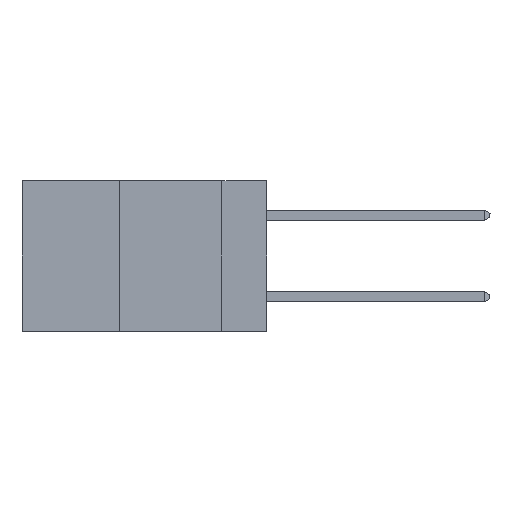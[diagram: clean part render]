
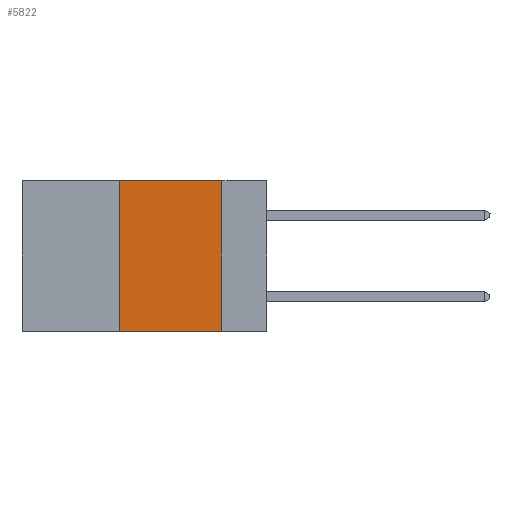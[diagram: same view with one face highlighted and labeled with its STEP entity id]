
A CAD part, left-side view. The second image highlights one B-rep face of the part: STEP entity #5822.
In plain terms, the highlighted planar face has unit normal (-1, 0, 0).
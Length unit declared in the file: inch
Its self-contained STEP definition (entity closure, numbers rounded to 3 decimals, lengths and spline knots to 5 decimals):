
#337 = DIRECTION ( 'NONE',  ( 0., -1., 0. ) ) ;
#737 = CARTESIAN_POINT ( 'NONE',  ( 0., 0.36, 0. ) ) ;
#1369 = LINE ( 'NONE', #12020, #12686 ) ;
#2554 = EDGE_CURVE ( 'NONE', #6572, #6282, #17058, .T. ) ;
#3341 = ORIENTED_EDGE ( 'NONE', *, *, #2554, .T. ) ;
#3881 = LINE ( 'NONE', #17930, #14264 ) ;
#4101 = CARTESIAN_POINT ( 'NONE',  ( 0., 0.36, 0. ) ) ;
#5822 = ADVANCED_FACE ( 'NONE', ( #9731 ), #19929, .F. ) ;
#5995 = EDGE_LOOP ( 'NONE', ( #15096, #18380, #22753, #3341 ) ) ;
#6282 = VERTEX_POINT ( 'NONE', #9473 ) ;
#6572 = VERTEX_POINT ( 'NONE', #19521 ) ;
#8205 = VECTOR ( 'NONE', #18675, 39.37008 ) ;
#8872 = EDGE_CURVE ( 'NONE', #9933, #14771, #3881, .T. ) ;
#9473 = CARTESIAN_POINT ( 'NONE',  ( 0., 0.11, -0.37 ) ) ;
#9731 = FACE_OUTER_BOUND ( 'NONE', #5995, .T. ) ;
#9933 = VERTEX_POINT ( 'NONE', #737 ) ;
#10208 = AXIS2_PLACEMENT_3D ( 'NONE', #21669, #11010, #18157 ) ;
#11010 = DIRECTION ( 'NONE',  ( 1., 0., 0. ) ) ;
#12020 = CARTESIAN_POINT ( 'NONE',  ( 0., 0.11, 0. ) ) ;
#12315 = VECTOR ( 'NONE', #20284, 39.37008 ) ;
#12686 = VECTOR ( 'NONE', #19186, 39.37008 ) ;
#13643 = CARTESIAN_POINT ( 'NONE',  ( 0., 0.6, -0.37 ) ) ;
#14264 = VECTOR ( 'NONE', #337, 39.37008 ) ;
#14379 = EDGE_CURVE ( 'NONE', #14771, #6282, #1369, .T. ) ;
#14771 = VERTEX_POINT ( 'NONE', #22022 ) ;
#15096 = ORIENTED_EDGE ( 'NONE', *, *, #14379, .F. ) ;
#17058 = LINE ( 'NONE', #13643, #8205 ) ;
#17930 = CARTESIAN_POINT ( 'NONE',  ( 0., 0.6, 0. ) ) ;
#18157 = DIRECTION ( 'NONE',  ( 0., 0., -1. ) ) ;
#18380 = ORIENTED_EDGE ( 'NONE', *, *, #8872, .F. ) ;
#18636 = LINE ( 'NONE', #4101, #12315 ) ;
#18675 = DIRECTION ( 'NONE',  ( 0., -1., 0. ) ) ;
#19186 = DIRECTION ( 'NONE',  ( 0., 0., -1. ) ) ;
#19521 = CARTESIAN_POINT ( 'NONE',  ( 0., 0.36, -0.37 ) ) ;
#19929 = PLANE ( 'NONE',  #10208 ) ;
#20284 = DIRECTION ( 'NONE',  ( 0., 0., 1. ) ) ;
#20800 = EDGE_CURVE ( 'NONE', #6572, #9933, #18636, .T. ) ;
#21669 = CARTESIAN_POINT ( 'NONE',  ( 0., 0.6, 0. ) ) ;
#22022 = CARTESIAN_POINT ( 'NONE',  ( 0., 0.11, 0. ) ) ;
#22753 = ORIENTED_EDGE ( 'NONE', *, *, #20800, .F. ) ;
